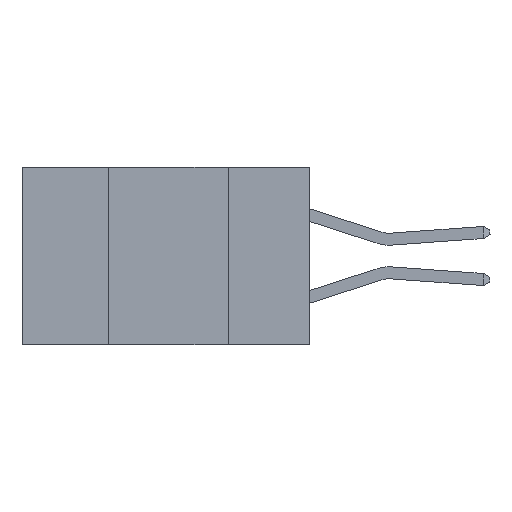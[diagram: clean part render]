
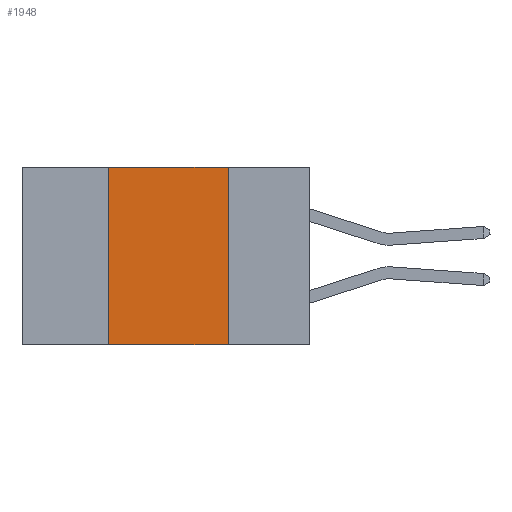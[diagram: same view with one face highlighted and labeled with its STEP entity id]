
A CAD part, left-side view. The second image highlights one B-rep face of the part: STEP entity #1948.
In plain terms, the highlighted planar face has unit normal (-1, 0, 0).
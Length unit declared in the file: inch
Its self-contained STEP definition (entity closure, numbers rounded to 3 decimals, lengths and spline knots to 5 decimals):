
#127 = CARTESIAN_POINT ( 'NONE',  ( 0., 0.17, -0.37 ) ) ;
#309 = VECTOR ( 'NONE', #9751, 39.37008 ) ;
#636 = LINE ( 'NONE', #2087, #309 ) ;
#1615 = FACE_OUTER_BOUND ( 'NONE', #8914, .T. ) ;
#1946 = VECTOR ( 'NONE', #5078, 39.37008 ) ;
#1948 = ADVANCED_FACE ( 'NONE', ( #1615 ), #3100, .F. ) ;
#2087 = CARTESIAN_POINT ( 'NONE',  ( 0., 0.6, 0. ) ) ;
#2460 = VERTEX_POINT ( 'NONE', #10934 ) ;
#2640 = VERTEX_POINT ( 'NONE', #10200 ) ;
#2698 = VECTOR ( 'NONE', #8263, 39.37008 ) ;
#2974 = EDGE_CURVE ( 'NONE', #2640, #2460, #10308, .T. ) ;
#3100 = PLANE ( 'NONE',  #4165 ) ;
#3215 = DIRECTION ( 'NONE',  ( 0., 0., -1. ) ) ;
#3243 = DIRECTION ( 'NONE',  ( 1., 0., 0. ) ) ;
#3244 = DIRECTION ( 'NONE',  ( 0., 0., -1. ) ) ;
#3421 = CARTESIAN_POINT ( 'NONE',  ( 0., 0.6, 0. ) ) ;
#4165 = AXIS2_PLACEMENT_3D ( 'NONE', #3421, #3243, #3215 ) ;
#4171 = CARTESIAN_POINT ( 'NONE',  ( 0., 0.17, -0.37 ) ) ;
#4499 = ORIENTED_EDGE ( 'NONE', *, *, #8239, .F. ) ;
#4558 = LINE ( 'NONE', #10746, #1946 ) ;
#4787 = ORIENTED_EDGE ( 'NONE', *, *, #2974, .F. ) ;
#5078 = DIRECTION ( 'NONE',  ( 0., -1., 0. ) ) ;
#5907 = LINE ( 'NONE', #4171, #10721 ) ;
#7525 = ORIENTED_EDGE ( 'NONE', *, *, #7590, .T. ) ;
#7590 = EDGE_CURVE ( 'NONE', #2640, #10618, #4558, .T. ) ;
#8211 = CARTESIAN_POINT ( 'NONE',  ( 0., 0.42, -0.37 ) ) ;
#8239 = EDGE_CURVE ( 'NONE', #2460, #9894, #636, .T. ) ;
#8263 = DIRECTION ( 'NONE',  ( 0., 0., 1. ) ) ;
#8914 = EDGE_LOOP ( 'NONE', ( #9214, #4499, #4787, #7525 ) ) ;
#9214 = ORIENTED_EDGE ( 'NONE', *, *, #10228, .F. ) ;
#9226 = CARTESIAN_POINT ( 'NONE',  ( 0., 0.17, 0. ) ) ;
#9751 = DIRECTION ( 'NONE',  ( 0., -1., 0. ) ) ;
#9894 = VERTEX_POINT ( 'NONE', #9226 ) ;
#10200 = CARTESIAN_POINT ( 'NONE',  ( 0., 0.42, -0.37 ) ) ;
#10228 = EDGE_CURVE ( 'NONE', #9894, #10618, #5907, .T. ) ;
#10308 = LINE ( 'NONE', #8211, #2698 ) ;
#10618 = VERTEX_POINT ( 'NONE', #127 ) ;
#10721 = VECTOR ( 'NONE', #3244, 39.37008 ) ;
#10746 = CARTESIAN_POINT ( 'NONE',  ( 0., 0.6, -0.37 ) ) ;
#10934 = CARTESIAN_POINT ( 'NONE',  ( 0., 0.42, 0. ) ) ;
